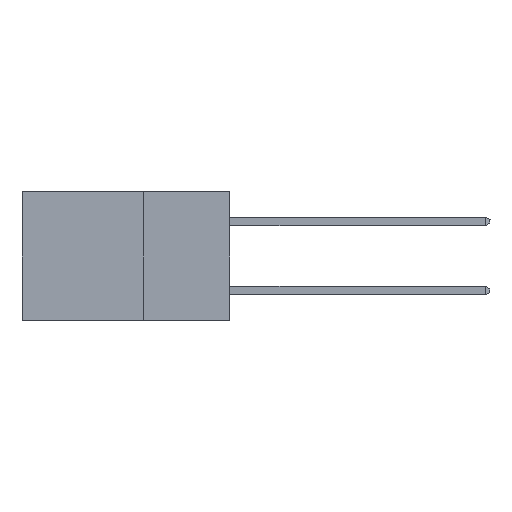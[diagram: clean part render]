
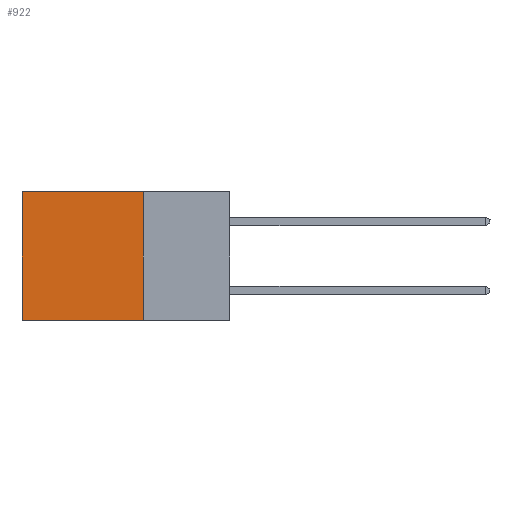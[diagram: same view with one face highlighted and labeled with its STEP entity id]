
A CAD part, left-side view. The second image highlights one B-rep face of the part: STEP entity #922.
In plain terms, the highlighted planar face has unit normal (-1, 0, 0).
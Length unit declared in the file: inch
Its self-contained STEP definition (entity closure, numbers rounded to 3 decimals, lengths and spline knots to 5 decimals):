
#922 = ADVANCED_FACE ( 'NONE', ( #5021 ), #12730, .F. ) ;
#1031 = VECTOR ( 'NONE', #24676, 39.37008 ) ;
#2295 = EDGE_CURVE ( 'NONE', #7063, #16257, #24865, .T. ) ;
#3071 = DIRECTION ( 'NONE',  ( 0., 1., 0. ) ) ;
#3112 = DIRECTION ( 'NONE',  ( 1., 0., 0. ) ) ;
#3435 = LINE ( 'NONE', #11158, #1031 ) ;
#3446 = CARTESIAN_POINT ( 'NONE',  ( 0.2615, 0.6, 0. ) ) ;
#4373 = CARTESIAN_POINT ( 'NONE',  ( 0.2615, 0.6, -0.37 ) ) ;
#4411 = ORIENTED_EDGE ( 'NONE', *, *, #7387, .F. ) ;
#4529 = AXIS2_PLACEMENT_3D ( 'NONE', #20434, #3112, #10844 ) ;
#5021 = FACE_OUTER_BOUND ( 'NONE', #19566, .T. ) ;
#5462 = LINE ( 'NONE', #20646, #23054 ) ;
#7063 = VERTEX_POINT ( 'NONE', #21902 ) ;
#7387 = EDGE_CURVE ( 'NONE', #7063, #14444, #3435, .T. ) ;
#10844 = DIRECTION ( 'NONE',  ( 0., 0., -1. ) ) ;
#11158 = CARTESIAN_POINT ( 'NONE',  ( 0.2615, 0.25, -0.37 ) ) ;
#11336 = VECTOR ( 'NONE', #17957, 39.37008 ) ;
#12730 = PLANE ( 'NONE',  #4529 ) ;
#13500 = DIRECTION ( 'NONE',  ( 0., 1., 0. ) ) ;
#14444 = VERTEX_POINT ( 'NONE', #19314 ) ;
#15412 = EDGE_CURVE ( 'NONE', #16257, #19208, #18075, .T. ) ;
#16242 = ORIENTED_EDGE ( 'NONE', *, *, #2295, .T. ) ;
#16257 = VERTEX_POINT ( 'NONE', #3446 ) ;
#16355 = EDGE_CURVE ( 'NONE', #14444, #19208, #5462, .T. ) ;
#17957 = DIRECTION ( 'NONE',  ( 0., 0., -1. ) ) ;
#18075 = LINE ( 'NONE', #18203, #11336 ) ;
#18203 = CARTESIAN_POINT ( 'NONE',  ( 0.2615, 0.6, -0.37 ) ) ;
#18283 = VECTOR ( 'NONE', #13500, 39.37008 ) ;
#19208 = VERTEX_POINT ( 'NONE', #4373 ) ;
#19314 = CARTESIAN_POINT ( 'NONE',  ( 0.2615, 0.25, -0.37 ) ) ;
#19566 = EDGE_LOOP ( 'NONE', ( #21658, #19717, #4411, #16242 ) ) ;
#19717 = ORIENTED_EDGE ( 'NONE', *, *, #16355, .F. ) ;
#20434 = CARTESIAN_POINT ( 'NONE',  ( 0.2615, 0.25, -0.37 ) ) ;
#20646 = CARTESIAN_POINT ( 'NONE',  ( 0.2615, 0.25, -0.37 ) ) ;
#21311 = CARTESIAN_POINT ( 'NONE',  ( 0.2615, 0.25, 0. ) ) ;
#21658 = ORIENTED_EDGE ( 'NONE', *, *, #15412, .T. ) ;
#21902 = CARTESIAN_POINT ( 'NONE',  ( 0.2615, 0.25, 0. ) ) ;
#23054 = VECTOR ( 'NONE', #3071, 39.37008 ) ;
#24676 = DIRECTION ( 'NONE',  ( 0., 0., -1. ) ) ;
#24865 = LINE ( 'NONE', #21311, #18283 ) ;
